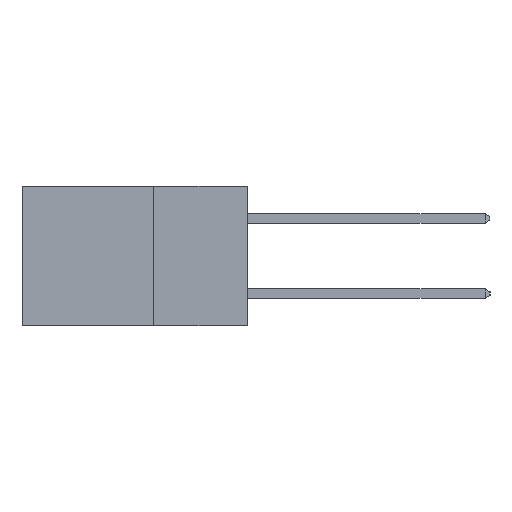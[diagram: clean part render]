
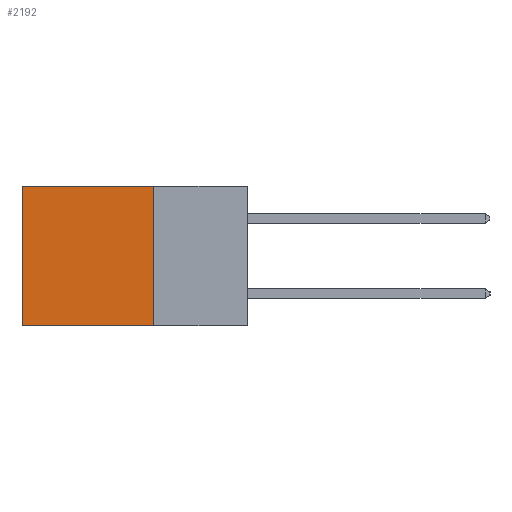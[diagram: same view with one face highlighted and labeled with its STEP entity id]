
A CAD part, left-side view. The second image highlights one B-rep face of the part: STEP entity #2192.
In plain terms, the highlighted planar face has unit normal (-1, 0, 0).
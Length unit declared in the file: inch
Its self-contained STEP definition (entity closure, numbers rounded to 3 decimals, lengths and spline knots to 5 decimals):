
#28 = LINE ( 'NONE', #11925, #12444 ) ;
#190 = EDGE_CURVE ( 'NONE', #9212, #15298, #28, .T. ) ;
#191 = LINE ( 'NONE', #6194, #6710 ) ;
#824 = AXIS2_PLACEMENT_3D ( 'NONE', #13297, #13190, #13091 ) ;
#955 = EDGE_CURVE ( 'NONE', #9212, #2114, #191, .T. ) ;
#1462 = LINE ( 'NONE', #3605, #11370 ) ;
#1502 = DIRECTION ( 'NONE',  ( 0., 1., 0. ) ) ;
#2114 = VERTEX_POINT ( 'NONE', #14930 ) ;
#2192 = ADVANCED_FACE ( 'NONE', ( #15671 ), #13204, .F. ) ;
#2459 = VERTEX_POINT ( 'NONE', #8710 ) ;
#2465 = LINE ( 'NONE', #15142, #12312 ) ;
#3605 = CARTESIAN_POINT ( 'NONE',  ( 0.2615, 0.6, -0.37 ) ) ;
#4158 = ORIENTED_EDGE ( 'NONE', *, *, #955, .T. ) ;
#5033 = ORIENTED_EDGE ( 'NONE', *, *, #9803, .F. ) ;
#6194 = CARTESIAN_POINT ( 'NONE',  ( 0.2615, 0.25, 0. ) ) ;
#6222 = CARTESIAN_POINT ( 'NONE',  ( 0.2615, 0.25, 0. ) ) ;
#6710 = VECTOR ( 'NONE', #1502, 39.37008 ) ;
#7609 = CARTESIAN_POINT ( 'NONE',  ( 0.2615, 0.25, -0.37 ) ) ;
#8676 = DIRECTION ( 'NONE',  ( 0., 0., -1. ) ) ;
#8710 = CARTESIAN_POINT ( 'NONE',  ( 0.2615, 0.6, -0.37 ) ) ;
#8830 = DIRECTION ( 'NONE',  ( 0., 0., -1. ) ) ;
#9204 = EDGE_CURVE ( 'NONE', #2114, #2459, #1462, .T. ) ;
#9212 = VERTEX_POINT ( 'NONE', #6222 ) ;
#9803 = EDGE_CURVE ( 'NONE', #15298, #2459, #2465, .T. ) ;
#10381 = ORIENTED_EDGE ( 'NONE', *, *, #190, .F. ) ;
#11179 = EDGE_LOOP ( 'NONE', ( #13284, #5033, #10381, #4158 ) ) ;
#11370 = VECTOR ( 'NONE', #8830, 39.37008 ) ;
#11398 = DIRECTION ( 'NONE',  ( 0., 1., 0. ) ) ;
#11925 = CARTESIAN_POINT ( 'NONE',  ( 0.2615, 0.25, -0.37 ) ) ;
#12312 = VECTOR ( 'NONE', #11398, 39.37008 ) ;
#12444 = VECTOR ( 'NONE', #8676, 39.37008 ) ;
#13091 = DIRECTION ( 'NONE',  ( 0., 0., -1. ) ) ;
#13190 = DIRECTION ( 'NONE',  ( 1., 0., 0. ) ) ;
#13204 = PLANE ( 'NONE',  #824 ) ;
#13284 = ORIENTED_EDGE ( 'NONE', *, *, #9204, .T. ) ;
#13297 = CARTESIAN_POINT ( 'NONE',  ( 0.2615, 0.25, -0.37 ) ) ;
#14930 = CARTESIAN_POINT ( 'NONE',  ( 0.2615, 0.6, 0. ) ) ;
#15142 = CARTESIAN_POINT ( 'NONE',  ( 0.2615, 0.25, -0.37 ) ) ;
#15298 = VERTEX_POINT ( 'NONE', #7609 ) ;
#15671 = FACE_OUTER_BOUND ( 'NONE', #11179, .T. ) ;
